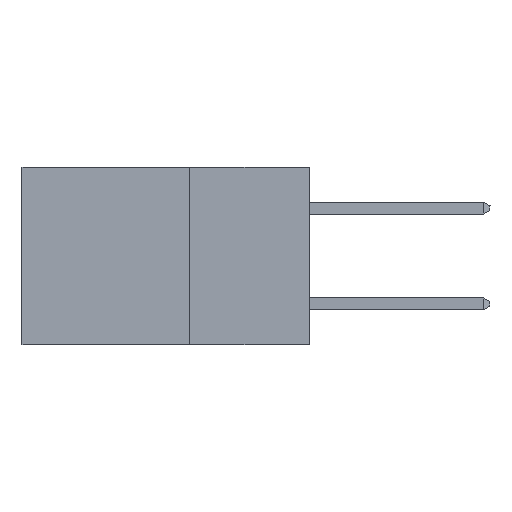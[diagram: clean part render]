
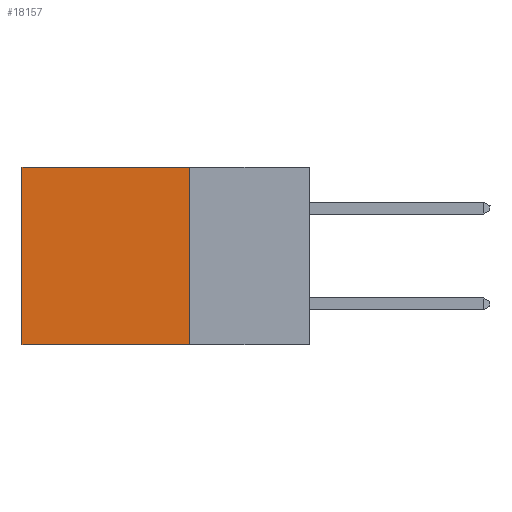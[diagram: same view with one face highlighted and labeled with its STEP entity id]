
A CAD part, left-side view. The second image highlights one B-rep face of the part: STEP entity #18157.
In plain terms, the highlighted planar face has unit normal (-1, 0, 0).
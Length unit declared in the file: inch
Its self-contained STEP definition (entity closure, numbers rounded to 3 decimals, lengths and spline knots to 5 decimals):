
#596 = VECTOR ( 'NONE', #5844, 39.37008 ) ;
#700 = VECTOR ( 'NONE', #18636, 39.37008 ) ;
#1460 = EDGE_CURVE ( 'NONE', #15663, #17432, #5321, .T. ) ;
#2123 = ORIENTED_EDGE ( 'NONE', *, *, #1460, .F. ) ;
#3435 = LINE ( 'NONE', #8444, #21349 ) ;
#3936 = EDGE_CURVE ( 'NONE', #17432, #10236, #4961, .T. ) ;
#4450 = CARTESIAN_POINT ( 'NONE',  ( 0.2875, 0.25, 0. ) ) ;
#4961 = LINE ( 'NONE', #10967, #596 ) ;
#5321 = LINE ( 'NONE', #8475, #700 ) ;
#5844 = DIRECTION ( 'NONE',  ( 0., 1., 0. ) ) ;
#6952 = CARTESIAN_POINT ( 'NONE',  ( 0.2875, 0.6, 0. ) ) ;
#7102 = VECTOR ( 'NONE', #12569, 39.37008 ) ;
#7780 = ORIENTED_EDGE ( 'NONE', *, *, #11789, .T. ) ;
#7785 = CARTESIAN_POINT ( 'NONE',  ( 0.2875, 0.25, -0.37 ) ) ;
#8444 = CARTESIAN_POINT ( 'NONE',  ( 0.2875, 0.25, 0. ) ) ;
#8475 = CARTESIAN_POINT ( 'NONE',  ( 0.2875, 0.25, 0. ) ) ;
#10236 = VERTEX_POINT ( 'NONE', #18221 ) ;
#10967 = CARTESIAN_POINT ( 'NONE',  ( 0.2875, 0.25, -0.37 ) ) ;
#11080 = DIRECTION ( 'NONE',  ( 1., 0., 0. ) ) ;
#11234 = CARTESIAN_POINT ( 'NONE',  ( 0.2875, 0.25, 0. ) ) ;
#11789 = EDGE_CURVE ( 'NONE', #18662, #10236, #14388, .T. ) ;
#12569 = DIRECTION ( 'NONE',  ( 0., 0., -1. ) ) ;
#13219 = ORIENTED_EDGE ( 'NONE', *, *, #15211, .T. ) ;
#14388 = LINE ( 'NONE', #16193, #7102 ) ;
#15211 = EDGE_CURVE ( 'NONE', #15663, #18662, #3435, .T. ) ;
#15663 = VERTEX_POINT ( 'NONE', #4450 ) ;
#16193 = CARTESIAN_POINT ( 'NONE',  ( 0.2875, 0.6, 0. ) ) ;
#16450 = AXIS2_PLACEMENT_3D ( 'NONE', #11234, #11080, #21761 ) ;
#17008 = DIRECTION ( 'NONE',  ( 0., 1., 0. ) ) ;
#17432 = VERTEX_POINT ( 'NONE', #7785 ) ;
#17559 = FACE_OUTER_BOUND ( 'NONE', #20528, .T. ) ;
#18157 = ADVANCED_FACE ( 'NONE', ( #17559 ), #21688, .F. ) ;
#18221 = CARTESIAN_POINT ( 'NONE',  ( 0.2875, 0.6, -0.37 ) ) ;
#18636 = DIRECTION ( 'NONE',  ( 0., 0., -1. ) ) ;
#18662 = VERTEX_POINT ( 'NONE', #6952 ) ;
#20528 = EDGE_LOOP ( 'NONE', ( #7780, #20616, #2123, #13219 ) ) ;
#20616 = ORIENTED_EDGE ( 'NONE', *, *, #3936, .F. ) ;
#21349 = VECTOR ( 'NONE', #17008, 39.37008 ) ;
#21688 = PLANE ( 'NONE',  #16450 ) ;
#21761 = DIRECTION ( 'NONE',  ( 0., 0., -1. ) ) ;
